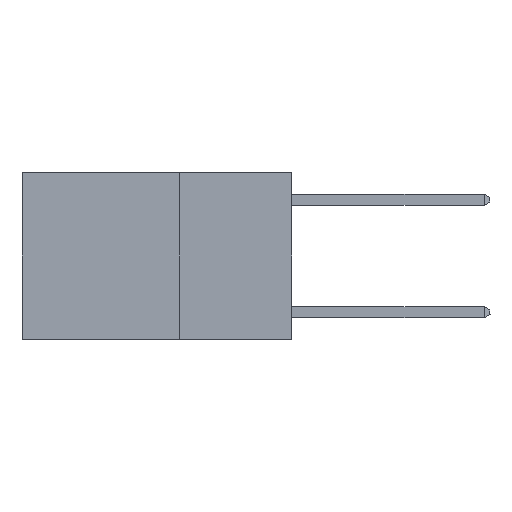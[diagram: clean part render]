
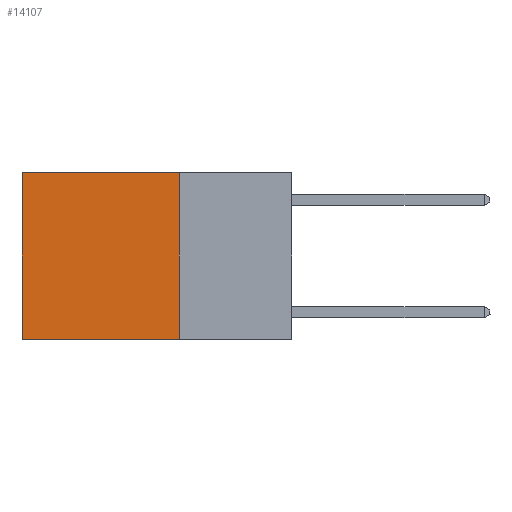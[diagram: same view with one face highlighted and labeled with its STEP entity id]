
A CAD part, left-side view. The second image highlights one B-rep face of the part: STEP entity #14107.
In plain terms, the highlighted planar face has unit normal (-1, 0, 0).
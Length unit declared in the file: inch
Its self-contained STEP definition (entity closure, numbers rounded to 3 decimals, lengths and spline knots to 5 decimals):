
#249 = CARTESIAN_POINT ( 'NONE',  ( 0.2625, 0.25, 0. ) ) ;
#1223 = ORIENTED_EDGE ( 'NONE', *, *, #1767, .F. ) ;
#1767 = EDGE_CURVE ( 'NONE', #9234, #24894, #10938, .T. ) ;
#2427 = DIRECTION ( 'NONE',  ( 0., 0., -1. ) ) ;
#4000 = LINE ( 'NONE', #4558, #21821 ) ;
#4487 = VECTOR ( 'NONE', #6900, 39.37008 ) ;
#4558 = CARTESIAN_POINT ( 'NONE',  ( 0.2625, 0.6, 0. ) ) ;
#6785 = DIRECTION ( 'NONE',  ( 0., 0., -1. ) ) ;
#6900 = DIRECTION ( 'NONE',  ( 0., 1., 0. ) ) ;
#7371 = CARTESIAN_POINT ( 'NONE',  ( 0.2625, 0.25, 0. ) ) ;
#7399 = ORIENTED_EDGE ( 'NONE', *, *, #25591, .T. ) ;
#7972 = EDGE_CURVE ( 'NONE', #14030, #16548, #9276, .T. ) ;
#9177 = CARTESIAN_POINT ( 'NONE',  ( 0.2625, 0.25, 0. ) ) ;
#9234 = VERTEX_POINT ( 'NONE', #11176 ) ;
#9276 = LINE ( 'NONE', #9177, #14615 ) ;
#9801 = CARTESIAN_POINT ( 'NONE',  ( 0.2625, 0.25, 0. ) ) ;
#9932 = ORIENTED_EDGE ( 'NONE', *, *, #7972, .T. ) ;
#10659 = EDGE_CURVE ( 'NONE', #14030, #9234, #25417, .T. ) ;
#10938 = LINE ( 'NONE', #21863, #4487 ) ;
#11176 = CARTESIAN_POINT ( 'NONE',  ( 0.2625, 0.25, -0.37 ) ) ;
#11343 = DIRECTION ( 'NONE',  ( 0., 1., 0. ) ) ;
#11723 = ORIENTED_EDGE ( 'NONE', *, *, #10659, .F. ) ;
#11970 = DIRECTION ( 'NONE',  ( 0., 0., -1. ) ) ;
#13518 = VECTOR ( 'NONE', #2427, 39.37008 ) ;
#14030 = VERTEX_POINT ( 'NONE', #7371 ) ;
#14107 = ADVANCED_FACE ( 'NONE', ( #24563 ), #18363, .F. ) ;
#14615 = VECTOR ( 'NONE', #11343, 39.37008 ) ;
#16548 = VERTEX_POINT ( 'NONE', #26078 ) ;
#18363 = PLANE ( 'NONE',  #22001 ) ;
#19765 = CARTESIAN_POINT ( 'NONE',  ( 0.2625, 0.6, -0.37 ) ) ;
#21821 = VECTOR ( 'NONE', #6785, 39.37008 ) ;
#21863 = CARTESIAN_POINT ( 'NONE',  ( 0.2625, 0.25, -0.37 ) ) ;
#22001 = AXIS2_PLACEMENT_3D ( 'NONE', #9801, #24658, #11970 ) ;
#22718 = EDGE_LOOP ( 'NONE', ( #7399, #1223, #11723, #9932 ) ) ;
#24563 = FACE_OUTER_BOUND ( 'NONE', #22718, .T. ) ;
#24658 = DIRECTION ( 'NONE',  ( 1., 0., 0. ) ) ;
#24894 = VERTEX_POINT ( 'NONE', #19765 ) ;
#25417 = LINE ( 'NONE', #249, #13518 ) ;
#25591 = EDGE_CURVE ( 'NONE', #16548, #24894, #4000, .T. ) ;
#26078 = CARTESIAN_POINT ( 'NONE',  ( 0.2625, 0.6, 0. ) ) ;
